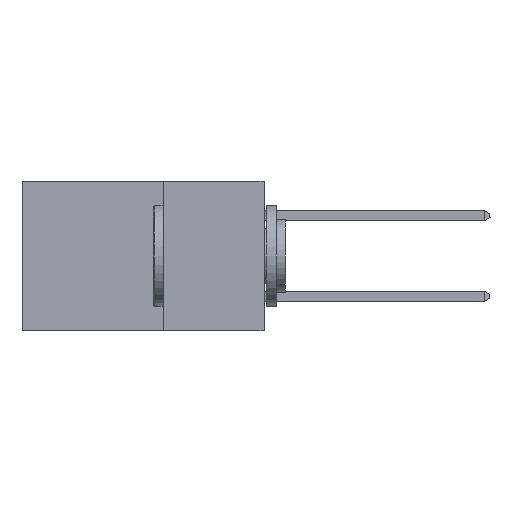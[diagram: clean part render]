
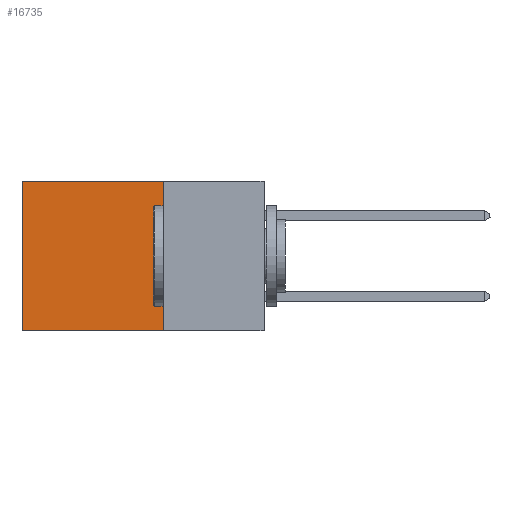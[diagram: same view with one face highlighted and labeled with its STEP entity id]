
A CAD part, left-side view. The second image highlights one B-rep face of the part: STEP entity #16735.
In plain terms, the highlighted planar face has unit normal (-1, 0, 0).
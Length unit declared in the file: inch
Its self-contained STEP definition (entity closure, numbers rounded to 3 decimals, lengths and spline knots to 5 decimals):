
#387 = EDGE_CURVE ( 'NONE', #7271, #5123, #17970, .T. ) ;
#483 = CARTESIAN_POINT ( 'NONE',  ( 0.298, 0.25, -0.37 ) ) ;
#1325 = DIRECTION ( 'NONE',  ( 0., 0., -1. ) ) ;
#1358 = VECTOR ( 'NONE', #8185, 39.37008 ) ;
#2867 = PLANE ( 'NONE',  #13417 ) ;
#3540 = DIRECTION ( 'NONE',  ( 0., 1., 0. ) ) ;
#3639 = ORIENTED_EDGE ( 'NONE', *, *, #387, .T. ) ;
#4503 = CARTESIAN_POINT ( 'NONE',  ( 0.298, 0.25, -0.37 ) ) ;
#5123 = VERTEX_POINT ( 'NONE', #9689 ) ;
#5544 = LINE ( 'NONE', #4503, #18144 ) ;
#6537 = ORIENTED_EDGE ( 'NONE', *, *, #9380, .F. ) ;
#6777 = CARTESIAN_POINT ( 'NONE',  ( 0.298, 0.25, 0. ) ) ;
#6803 = LINE ( 'NONE', #12913, #1358 ) ;
#7271 = VERTEX_POINT ( 'NONE', #6777 ) ;
#8185 = DIRECTION ( 'NONE',  ( 0., 0., -1. ) ) ;
#8237 = CARTESIAN_POINT ( 'NONE',  ( 0.298, 0.6, -0.37 ) ) ;
#8322 = EDGE_LOOP ( 'NONE', ( #14244, #13193, #6537, #3639 ) ) ;
#8990 = VECTOR ( 'NONE', #3540, 39.37008 ) ;
#9177 = LINE ( 'NONE', #19240, #12711 ) ;
#9380 = EDGE_CURVE ( 'NONE', #7271, #15799, #9177, .T. ) ;
#9467 = VERTEX_POINT ( 'NONE', #8237 ) ;
#9689 = CARTESIAN_POINT ( 'NONE',  ( 0.298, 0.6, 0. ) ) ;
#10152 = DIRECTION ( 'NONE',  ( 0., 0., -1. ) ) ;
#12711 = VECTOR ( 'NONE', #10152, 39.37008 ) ;
#12913 = CARTESIAN_POINT ( 'NONE',  ( 0.298, 0.6, 0. ) ) ;
#13193 = ORIENTED_EDGE ( 'NONE', *, *, #16054, .F. ) ;
#13417 = AXIS2_PLACEMENT_3D ( 'NONE', #13500, #15199, #1325 ) ;
#13500 = CARTESIAN_POINT ( 'NONE',  ( 0.298, 0.25, 0. ) ) ;
#14016 = EDGE_CURVE ( 'NONE', #5123, #9467, #6803, .T. ) ;
#14244 = ORIENTED_EDGE ( 'NONE', *, *, #14016, .T. ) ;
#15199 = DIRECTION ( 'NONE',  ( 1., 0., 0. ) ) ;
#15567 = CARTESIAN_POINT ( 'NONE',  ( 0.298, 0.25, 0. ) ) ;
#15799 = VERTEX_POINT ( 'NONE', #483 ) ;
#16054 = EDGE_CURVE ( 'NONE', #15799, #9467, #5544, .T. ) ;
#16735 = ADVANCED_FACE ( 'NONE', ( #18344 ), #2867, .F. ) ;
#17970 = LINE ( 'NONE', #15567, #8990 ) ;
#18144 = VECTOR ( 'NONE', #19490, 39.37008 ) ;
#18344 = FACE_OUTER_BOUND ( 'NONE', #8322, .T. ) ;
#19240 = CARTESIAN_POINT ( 'NONE',  ( 0.298, 0.25, 0. ) ) ;
#19490 = DIRECTION ( 'NONE',  ( 0., 1., 0. ) ) ;
